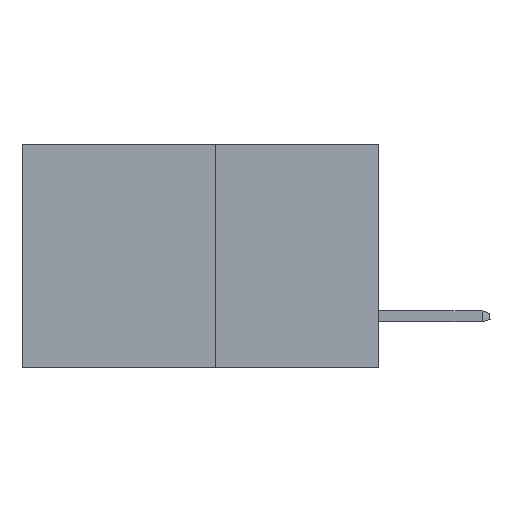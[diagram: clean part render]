
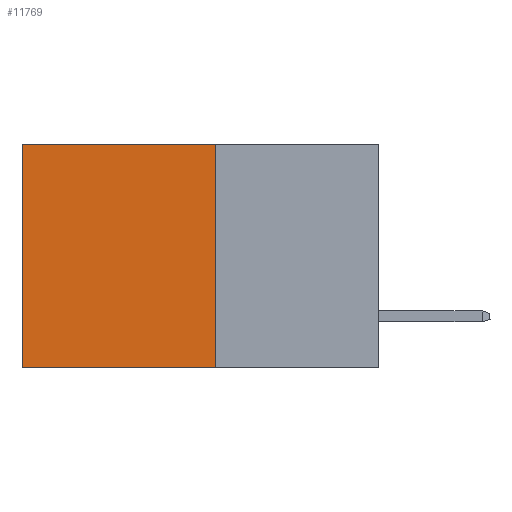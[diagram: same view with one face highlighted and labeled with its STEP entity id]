
A CAD part, left-side view. The second image highlights one B-rep face of the part: STEP entity #11769.
In plain terms, the highlighted planar face has unit normal (-1, 0, 0).
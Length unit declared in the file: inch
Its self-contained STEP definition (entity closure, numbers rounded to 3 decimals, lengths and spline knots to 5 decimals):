
#1104 = CARTESIAN_POINT ( 'NONE',  ( 0.277, 0.27, 0. ) ) ;
#1274 = VECTOR ( 'NONE', #13206, 39.37008 ) ;
#1933 = CARTESIAN_POINT ( 'NONE',  ( 0.277, 0.27, 0. ) ) ;
#2132 = ORIENTED_EDGE ( 'NONE', *, *, #22178, .T. ) ;
#2189 = CARTESIAN_POINT ( 'NONE',  ( 0.277, 0.59, -0.37 ) ) ;
#2934 = CARTESIAN_POINT ( 'NONE',  ( 0.277, 0.59, 0. ) ) ;
#3131 = DIRECTION ( 'NONE',  ( 0., 1., 0. ) ) ;
#4323 = VERTEX_POINT ( 'NONE', #17500 ) ;
#4860 = EDGE_LOOP ( 'NONE', ( #2132, #13804, #12419, #14378 ) ) ;
#5270 = EDGE_CURVE ( 'NONE', #11330, #8669, #10598, .T. ) ;
#6375 = DIRECTION ( 'NONE',  ( 0., 1., 0. ) ) ;
#8138 = PLANE ( 'NONE',  #12612 ) ;
#8669 = VERTEX_POINT ( 'NONE', #2934 ) ;
#8935 = LINE ( 'NONE', #10083, #13173 ) ;
#9865 = CARTESIAN_POINT ( 'NONE',  ( 0.277, 0.27, -0.37 ) ) ;
#9988 = DIRECTION ( 'NONE',  ( 0., 0., -1. ) ) ;
#10083 = CARTESIAN_POINT ( 'NONE',  ( 0.277, 0.27, -0.37 ) ) ;
#10598 = LINE ( 'NONE', #1933, #19448 ) ;
#11259 = EDGE_CURVE ( 'NONE', #4323, #12127, #8935, .T. ) ;
#11330 = VERTEX_POINT ( 'NONE', #1104 ) ;
#11769 = ADVANCED_FACE ( 'NONE', ( #21340 ), #8138, .F. ) ;
#12127 = VERTEX_POINT ( 'NONE', #23140 ) ;
#12419 = ORIENTED_EDGE ( 'NONE', *, *, #22823, .F. ) ;
#12612 = AXIS2_PLACEMENT_3D ( 'NONE', #15309, #20569, #9988 ) ;
#13173 = VECTOR ( 'NONE', #6375, 39.37008 ) ;
#13206 = DIRECTION ( 'NONE',  ( 0., 0., -1. ) ) ;
#13804 = ORIENTED_EDGE ( 'NONE', *, *, #11259, .F. ) ;
#14378 = ORIENTED_EDGE ( 'NONE', *, *, #5270, .T. ) ;
#14427 = VECTOR ( 'NONE', #20521, 39.37008 ) ;
#15309 = CARTESIAN_POINT ( 'NONE',  ( 0.277, 0.27, -0.37 ) ) ;
#15838 = LINE ( 'NONE', #2189, #1274 ) ;
#17500 = CARTESIAN_POINT ( 'NONE',  ( 0.277, 0.27, -0.37 ) ) ;
#19104 = LINE ( 'NONE', #9865, #14427 ) ;
#19448 = VECTOR ( 'NONE', #3131, 39.37008 ) ;
#20521 = DIRECTION ( 'NONE',  ( 0., 0., -1. ) ) ;
#20569 = DIRECTION ( 'NONE',  ( 1., 0., 0. ) ) ;
#21340 = FACE_OUTER_BOUND ( 'NONE', #4860, .T. ) ;
#22178 = EDGE_CURVE ( 'NONE', #8669, #12127, #15838, .T. ) ;
#22823 = EDGE_CURVE ( 'NONE', #11330, #4323, #19104, .T. ) ;
#23140 = CARTESIAN_POINT ( 'NONE',  ( 0.277, 0.59, -0.37 ) ) ;
